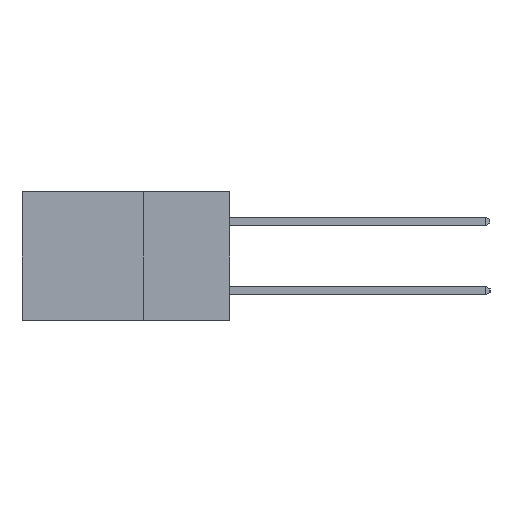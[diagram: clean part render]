
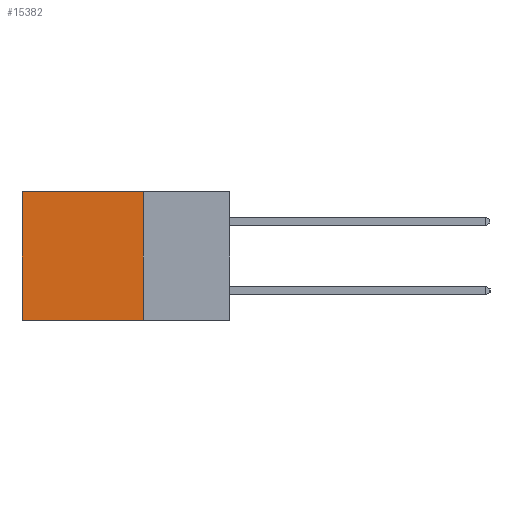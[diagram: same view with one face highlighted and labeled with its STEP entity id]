
A CAD part, left-side view. The second image highlights one B-rep face of the part: STEP entity #15382.
In plain terms, the highlighted planar face has unit normal (-1, 0, 0).
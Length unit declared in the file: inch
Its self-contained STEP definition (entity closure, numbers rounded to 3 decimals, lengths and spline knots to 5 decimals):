
#563 = ORIENTED_EDGE ( 'NONE', *, *, #7269, .F. ) ;
#852 = CARTESIAN_POINT ( 'NONE',  ( 0.2615, 0.25, -0.37 ) ) ;
#953 = LINE ( 'NONE', #13901, #7124 ) ;
#1453 = CARTESIAN_POINT ( 'NONE',  ( 0.2615, 0.25, -0.37 ) ) ;
#1520 = VERTEX_POINT ( 'NONE', #14920 ) ;
#1885 = ORIENTED_EDGE ( 'NONE', *, *, #17072, .T. ) ;
#2225 = DIRECTION ( 'NONE',  ( 0., 1., 0. ) ) ;
#2691 = CARTESIAN_POINT ( 'NONE',  ( 0.2615, 0.6, 0. ) ) ;
#2877 = PLANE ( 'NONE',  #12283 ) ;
#3149 = ORIENTED_EDGE ( 'NONE', *, *, #16464, .T. ) ;
#3817 = CARTESIAN_POINT ( 'NONE',  ( 0.2615, 0.25, 0. ) ) ;
#3961 = DIRECTION ( 'NONE',  ( 0., 0., -1. ) ) ;
#3998 = VERTEX_POINT ( 'NONE', #10785 ) ;
#5227 = DIRECTION ( 'NONE',  ( 0., 1., 0. ) ) ;
#5647 = EDGE_LOOP ( 'NONE', ( #3149, #563, #10843, #1885 ) ) ;
#5798 = LINE ( 'NONE', #852, #16399 ) ;
#6203 = VERTEX_POINT ( 'NONE', #12746 ) ;
#6841 = EDGE_CURVE ( 'NONE', #6203, #3998, #953, .T. ) ;
#6851 = LINE ( 'NONE', #3817, #17613 ) ;
#6905 = LINE ( 'NONE', #10953, #17480 ) ;
#7124 = VECTOR ( 'NONE', #15271, 39.37008 ) ;
#7269 = EDGE_CURVE ( 'NONE', #3998, #1520, #5798, .T. ) ;
#10452 = FACE_OUTER_BOUND ( 'NONE', #5647, .T. ) ;
#10785 = CARTESIAN_POINT ( 'NONE',  ( 0.2615, 0.25, -0.37 ) ) ;
#10843 = ORIENTED_EDGE ( 'NONE', *, *, #6841, .F. ) ;
#10953 = CARTESIAN_POINT ( 'NONE',  ( 0.2615, 0.6, -0.37 ) ) ;
#12283 = AXIS2_PLACEMENT_3D ( 'NONE', #1453, #16704, #12680 ) ;
#12680 = DIRECTION ( 'NONE',  ( 0., 0., -1. ) ) ;
#12746 = CARTESIAN_POINT ( 'NONE',  ( 0.2615, 0.25, 0. ) ) ;
#13901 = CARTESIAN_POINT ( 'NONE',  ( 0.2615, 0.25, -0.37 ) ) ;
#14920 = CARTESIAN_POINT ( 'NONE',  ( 0.2615, 0.6, -0.37 ) ) ;
#15271 = DIRECTION ( 'NONE',  ( 0., 0., -1. ) ) ;
#15382 = ADVANCED_FACE ( 'NONE', ( #10452 ), #2877, .F. ) ;
#16399 = VECTOR ( 'NONE', #2225, 39.37008 ) ;
#16464 = EDGE_CURVE ( 'NONE', #17223, #1520, #6905, .T. ) ;
#16704 = DIRECTION ( 'NONE',  ( 1., 0., 0. ) ) ;
#17072 = EDGE_CURVE ( 'NONE', #6203, #17223, #6851, .T. ) ;
#17223 = VERTEX_POINT ( 'NONE', #2691 ) ;
#17480 = VECTOR ( 'NONE', #3961, 39.37008 ) ;
#17613 = VECTOR ( 'NONE', #5227, 39.37008 ) ;
